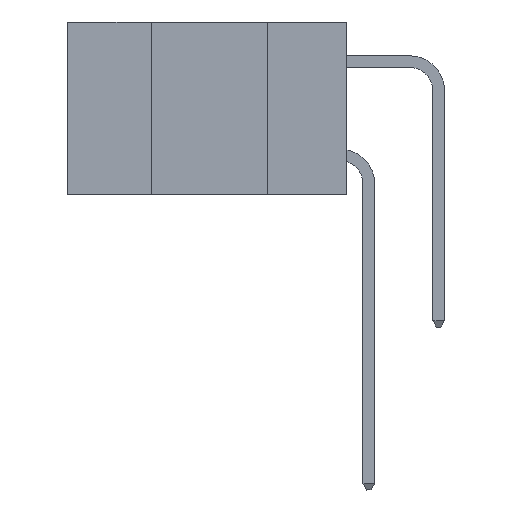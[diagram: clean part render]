
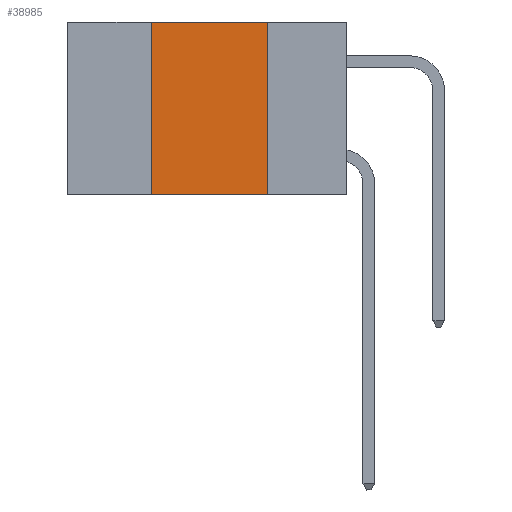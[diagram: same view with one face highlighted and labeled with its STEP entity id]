
A CAD part, left-side view. The second image highlights one B-rep face of the part: STEP entity #38985.
In plain terms, the highlighted planar face has unit normal (-1, 0, 0).
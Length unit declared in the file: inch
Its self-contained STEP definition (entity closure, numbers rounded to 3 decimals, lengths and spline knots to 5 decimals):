
#1015 = EDGE_CURVE ( 'NONE', #2011, #23943, #15305, .T. ) ;
#1351 = DIRECTION ( 'NONE',  ( 0., 0., -1. ) ) ;
#2011 = VERTEX_POINT ( 'NONE', #5886 ) ;
#3572 = VERTEX_POINT ( 'NONE', #26703 ) ;
#4333 = EDGE_CURVE ( 'NONE', #3572, #2011, #34334, .T. ) ;
#5876 = DIRECTION ( 'NONE',  ( 0., -1., 0. ) ) ;
#5886 = CARTESIAN_POINT ( 'NONE',  ( 0., 0.42, 0. ) ) ;
#6349 = DIRECTION ( 'NONE',  ( 0., -1., 0. ) ) ;
#7661 = CARTESIAN_POINT ( 'NONE',  ( 0., 0.17, -0.37 ) ) ;
#8270 = PLANE ( 'NONE',  #33270 ) ;
#10814 = VECTOR ( 'NONE', #6349, 39.37008 ) ;
#12347 = LINE ( 'NONE', #29233, #10814 ) ;
#12539 = CARTESIAN_POINT ( 'NONE',  ( 0., 0.6, 0. ) ) ;
#13506 = VERTEX_POINT ( 'NONE', #7661 ) ;
#14334 = CARTESIAN_POINT ( 'NONE',  ( 0., 0.6, 0. ) ) ;
#15263 = ORIENTED_EDGE ( 'NONE', *, *, #41198, .T. ) ;
#15305 = LINE ( 'NONE', #12539, #31469 ) ;
#17606 = DIRECTION ( 'NONE',  ( 1., 0., 0. ) ) ;
#17726 = ORIENTED_EDGE ( 'NONE', *, *, #4333, .F. ) ;
#23943 = VERTEX_POINT ( 'NONE', #30232 ) ;
#25127 = LINE ( 'NONE', #31834, #28652 ) ;
#25770 = VECTOR ( 'NONE', #28003, 39.37008 ) ;
#26703 = CARTESIAN_POINT ( 'NONE',  ( 0., 0.42, -0.37 ) ) ;
#27209 = FACE_OUTER_BOUND ( 'NONE', #38934, .T. ) ;
#28003 = DIRECTION ( 'NONE',  ( 0., 0., 1. ) ) ;
#28652 = VECTOR ( 'NONE', #31976, 39.37008 ) ;
#29026 = ORIENTED_EDGE ( 'NONE', *, *, #1015, .F. ) ;
#29233 = CARTESIAN_POINT ( 'NONE',  ( 0., 0.6, -0.37 ) ) ;
#30174 = CARTESIAN_POINT ( 'NONE',  ( 0., 0.42, 0. ) ) ;
#30232 = CARTESIAN_POINT ( 'NONE',  ( 0., 0.17, 0. ) ) ;
#31469 = VECTOR ( 'NONE', #5876, 39.37008 ) ;
#31834 = CARTESIAN_POINT ( 'NONE',  ( 0., 0.17, 0. ) ) ;
#31976 = DIRECTION ( 'NONE',  ( 0., 0., -1. ) ) ;
#32823 = EDGE_CURVE ( 'NONE', #23943, #13506, #25127, .T. ) ;
#33270 = AXIS2_PLACEMENT_3D ( 'NONE', #14334, #17606, #1351 ) ;
#34214 = ORIENTED_EDGE ( 'NONE', *, *, #32823, .F. ) ;
#34334 = LINE ( 'NONE', #30174, #25770 ) ;
#38934 = EDGE_LOOP ( 'NONE', ( #34214, #29026, #17726, #15263 ) ) ;
#38985 = ADVANCED_FACE ( 'NONE', ( #27209 ), #8270, .F. ) ;
#41198 = EDGE_CURVE ( 'NONE', #3572, #13506, #12347, .T. ) ;
